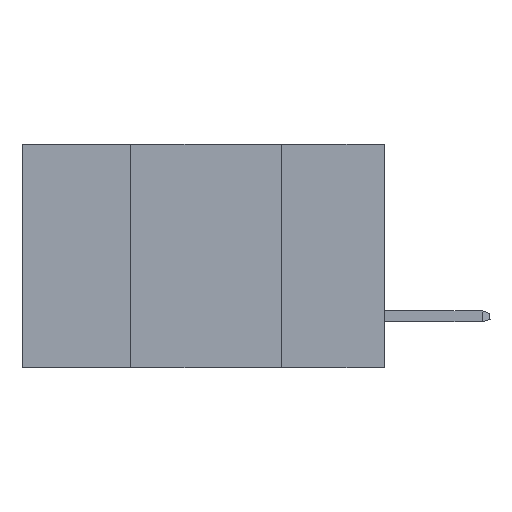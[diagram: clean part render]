
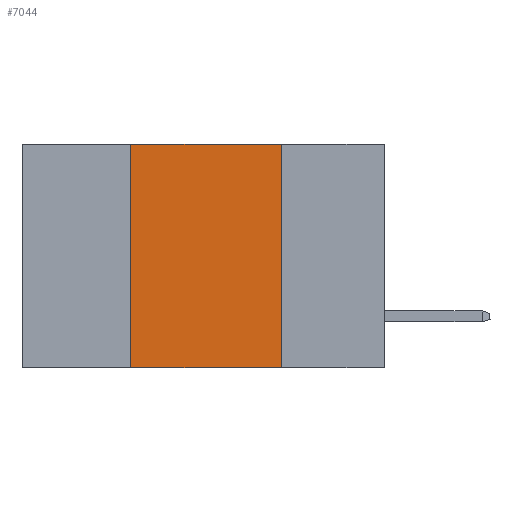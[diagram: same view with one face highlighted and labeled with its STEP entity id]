
A CAD part, left-side view. The second image highlights one B-rep face of the part: STEP entity #7044.
In plain terms, the highlighted planar face has unit normal (-1, 0, 0).
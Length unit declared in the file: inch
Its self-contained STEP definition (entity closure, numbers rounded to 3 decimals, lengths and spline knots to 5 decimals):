
#88 = DIRECTION ( 'NONE',  ( 0., 0., -1. ) ) ;
#548 = CARTESIAN_POINT ( 'NONE',  ( 0., 0.42, -0.37 ) ) ;
#675 = ORIENTED_EDGE ( 'NONE', *, *, #11173, .F. ) ;
#856 = CARTESIAN_POINT ( 'NONE',  ( 0., 0.42, 0. ) ) ;
#892 = VERTEX_POINT ( 'NONE', #2957 ) ;
#971 = VECTOR ( 'NONE', #15432, 39.37008 ) ;
#1525 = LINE ( 'NONE', #14569, #8240 ) ;
#1579 = CARTESIAN_POINT ( 'NONE',  ( 0., 0.17, -0.37 ) ) ;
#2237 = PLANE ( 'NONE',  #4772 ) ;
#2957 = CARTESIAN_POINT ( 'NONE',  ( 0., 0.17, 0. ) ) ;
#3066 = LINE ( 'NONE', #856, #5893 ) ;
#3158 = EDGE_CURVE ( 'NONE', #6663, #11920, #1525, .T. ) ;
#3994 = LINE ( 'NONE', #7058, #971 ) ;
#4643 = CARTESIAN_POINT ( 'NONE',  ( 0., 0.6, 0. ) ) ;
#4772 = AXIS2_PLACEMENT_3D ( 'NONE', #4643, #7108, #88 ) ;
#5272 = ORIENTED_EDGE ( 'NONE', *, *, #6791, .F. ) ;
#5893 = VECTOR ( 'NONE', #12816, 39.37008 ) ;
#6415 = VERTEX_POINT ( 'NONE', #8411 ) ;
#6663 = VERTEX_POINT ( 'NONE', #548 ) ;
#6791 = EDGE_CURVE ( 'NONE', #6663, #6415, #3066, .T. ) ;
#7044 = ADVANCED_FACE ( 'NONE', ( #10060 ), #2237, .F. ) ;
#7058 = CARTESIAN_POINT ( 'NONE',  ( 0., 0.17, 0. ) ) ;
#7108 = DIRECTION ( 'NONE',  ( 1., 0., 0. ) ) ;
#7293 = CARTESIAN_POINT ( 'NONE',  ( 0., 0.6, 0. ) ) ;
#8240 = VECTOR ( 'NONE', #13757, 39.37008 ) ;
#8411 = CARTESIAN_POINT ( 'NONE',  ( 0., 0.42, 0. ) ) ;
#8481 = LINE ( 'NONE', #7293, #12940 ) ;
#10060 = FACE_OUTER_BOUND ( 'NONE', #11137, .T. ) ;
#10485 = ORIENTED_EDGE ( 'NONE', *, *, #3158, .T. ) ;
#11004 = EDGE_CURVE ( 'NONE', #6415, #892, #8481, .T. ) ;
#11137 = EDGE_LOOP ( 'NONE', ( #675, #14851, #5272, #10485 ) ) ;
#11173 = EDGE_CURVE ( 'NONE', #892, #11920, #3994, .T. ) ;
#11920 = VERTEX_POINT ( 'NONE', #1579 ) ;
#12816 = DIRECTION ( 'NONE',  ( 0., 0., 1. ) ) ;
#12940 = VECTOR ( 'NONE', #14263, 39.37008 ) ;
#13757 = DIRECTION ( 'NONE',  ( 0., -1., 0. ) ) ;
#14263 = DIRECTION ( 'NONE',  ( 0., -1., 0. ) ) ;
#14569 = CARTESIAN_POINT ( 'NONE',  ( 0., 0.6, -0.37 ) ) ;
#14851 = ORIENTED_EDGE ( 'NONE', *, *, #11004, .F. ) ;
#15432 = DIRECTION ( 'NONE',  ( 0., 0., -1. ) ) ;
